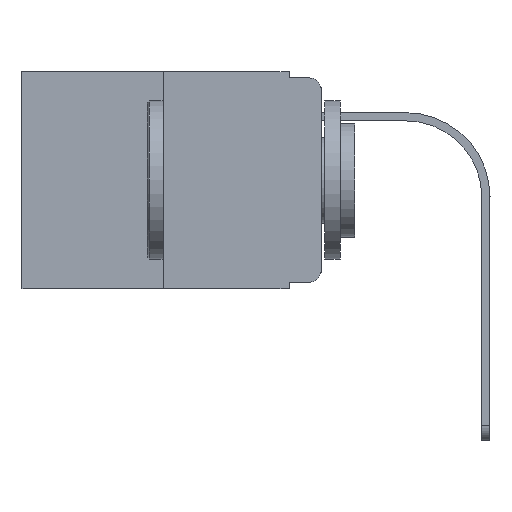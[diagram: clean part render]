
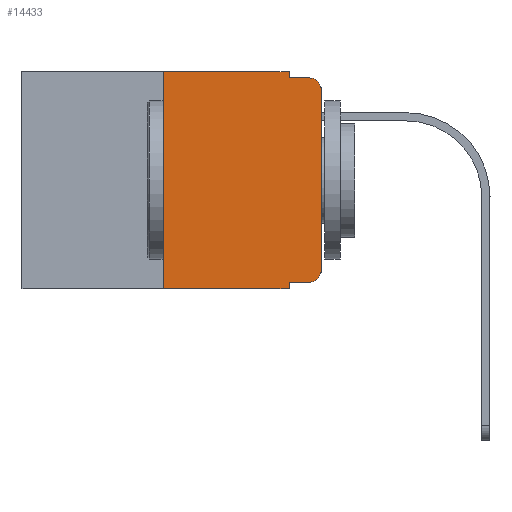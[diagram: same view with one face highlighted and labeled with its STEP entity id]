
A CAD part, left-side view. The second image highlights one B-rep face of the part: STEP entity #14433.
In plain terms, the highlighted planar face has unit normal (-1, 0, 0).
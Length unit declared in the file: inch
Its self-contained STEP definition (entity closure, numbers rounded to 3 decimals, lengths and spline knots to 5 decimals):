
#186 = CARTESIAN_POINT ( 'NONE',  ( 0., 0.051, -0.01 ) ) ;
#334 = CARTESIAN_POINT ( 'NONE',  ( 0., 0.02, -0.333 ) ) ;
#567 = DIRECTION ( 'NONE',  ( 0., -1., 0. ) ) ;
#605 = VECTOR ( 'NONE', #6141, 39.37008 ) ;
#712 = AXIS2_PLACEMENT_3D ( 'NONE', #1798, #9189, #21555 ) ;
#1086 = EDGE_CURVE ( 'NONE', #19642, #6668, #23073, .T. ) ;
#1165 = CARTESIAN_POINT ( 'NONE',  ( 0., 0.051, -0.01 ) ) ;
#1309 = CARTESIAN_POINT ( 'NONE',  ( 0., 0., -0.03 ) ) ;
#1361 = LINE ( 'NONE', #8524, #14861 ) ;
#1400 = ORIENTED_EDGE ( 'NONE', *, *, #13498, .F. ) ;
#1798 = CARTESIAN_POINT ( 'NONE',  ( 0., 0.02, -0.313 ) ) ;
#1829 = ORIENTED_EDGE ( 'NONE', *, *, #3514, .F. ) ;
#1975 = CARTESIAN_POINT ( 'NONE',  ( 0., 0.473, 0. ) ) ;
#2199 = EDGE_LOOP ( 'NONE', ( #4130, #20271, #1400, #1829, #14284, #20652, #4712, #16064, #18533, #12372 ) ) ;
#2959 = EDGE_CURVE ( 'NONE', #8968, #9520, #14927, .T. ) ;
#2961 = VECTOR ( 'NONE', #12769, 39.37008 ) ;
#3514 = EDGE_CURVE ( 'NONE', #9520, #6218, #1361, .T. ) ;
#3970 = CARTESIAN_POINT ( 'NONE',  ( 0., 0., 0. ) ) ;
#4130 = ORIENTED_EDGE ( 'NONE', *, *, #22395, .T. ) ;
#4528 = DIRECTION ( 'NONE',  ( 0., -1., 0. ) ) ;
#4606 = CARTESIAN_POINT ( 'NONE',  ( 0., 0.25, 0. ) ) ;
#4712 = ORIENTED_EDGE ( 'NONE', *, *, #4768, .T. ) ;
#4768 = EDGE_CURVE ( 'NONE', #12555, #6668, #19018, .T. ) ;
#5191 = EDGE_CURVE ( 'NONE', #19642, #13134, #20278, .T. ) ;
#6141 = DIRECTION ( 'NONE',  ( 0., -1., 0. ) ) ;
#6218 = VERTEX_POINT ( 'NONE', #1165 ) ;
#6524 = EDGE_CURVE ( 'NONE', #12555, #8968, #18800, .T. ) ;
#6668 = VERTEX_POINT ( 'NONE', #8411 ) ;
#6980 = DIRECTION ( 'NONE',  ( 0., 0., -1. ) ) ;
#7184 = DIRECTION ( 'NONE',  ( -1., 0., 0. ) ) ;
#7277 = FACE_OUTER_BOUND ( 'NONE', #2199, .T. ) ;
#8179 = CARTESIAN_POINT ( 'NONE',  ( 0., 0.473, -0.343 ) ) ;
#8202 = CIRCLE ( 'NONE', #11641, 0.02 ) ;
#8411 = CARTESIAN_POINT ( 'NONE',  ( 0., 0.051, -0.343 ) ) ;
#8524 = CARTESIAN_POINT ( 'NONE',  ( 0., 0.051, 0. ) ) ;
#8930 = CARTESIAN_POINT ( 'NONE',  ( 0., 0., -0.313 ) ) ;
#8968 = VERTEX_POINT ( 'NONE', #4606 ) ;
#9189 = DIRECTION ( 'NONE',  ( -1., 0., 0. ) ) ;
#9279 = DIRECTION ( 'NONE',  ( 0., 0., 1. ) ) ;
#9285 = PLANE ( 'NONE',  #16144 ) ;
#9520 = VERTEX_POINT ( 'NONE', #14572 ) ;
#10049 = CARTESIAN_POINT ( 'NONE',  ( 0., 0.25, -0.343 ) ) ;
#10499 = CARTESIAN_POINT ( 'NONE',  ( 0., 0.02, -0.03 ) ) ;
#11586 = CIRCLE ( 'NONE', #712, 0.02 ) ;
#11641 = AXIS2_PLACEMENT_3D ( 'NONE', #10499, #7184, #18031 ) ;
#12368 = DIRECTION ( 'NONE',  ( 0., 0., -1. ) ) ;
#12372 = ORIENTED_EDGE ( 'NONE', *, *, #19283, .T. ) ;
#12384 = DIRECTION ( 'NONE',  ( 0., 0., 1. ) ) ;
#12472 = CARTESIAN_POINT ( 'NONE',  ( 0., 0.051, -0.333 ) ) ;
#12555 = VERTEX_POINT ( 'NONE', #10049 ) ;
#12769 = DIRECTION ( 'NONE',  ( 0., -1., 0. ) ) ;
#12990 = LINE ( 'NONE', #186, #2961 ) ;
#13134 = VERTEX_POINT ( 'NONE', #334 ) ;
#13498 = EDGE_CURVE ( 'NONE', #6218, #17794, #12990, .T. ) ;
#13839 = CARTESIAN_POINT ( 'NONE',  ( 0., 0.25, 0. ) ) ;
#14284 = ORIENTED_EDGE ( 'NONE', *, *, #2959, .F. ) ;
#14433 = ADVANCED_FACE ( 'NONE', ( #7277 ), #9285, .F. ) ;
#14572 = CARTESIAN_POINT ( 'NONE',  ( 0., 0.051, 0. ) ) ;
#14861 = VECTOR ( 'NONE', #6980, 39.37008 ) ;
#14927 = LINE ( 'NONE', #1975, #16124 ) ;
#15494 = VECTOR ( 'NONE', #12384, 39.37008 ) ;
#15505 = DIRECTION ( 'NONE',  ( 1., 0., 0. ) ) ;
#15706 = VECTOR ( 'NONE', #12368, 39.37008 ) ;
#16064 = ORIENTED_EDGE ( 'NONE', *, *, #1086, .F. ) ;
#16124 = VECTOR ( 'NONE', #567, 39.37008 ) ;
#16144 = AXIS2_PLACEMENT_3D ( 'NONE', #19155, #15505, #22570 ) ;
#17794 = VERTEX_POINT ( 'NONE', #19221 ) ;
#18031 = DIRECTION ( 'NONE',  ( 0., 0., -1. ) ) ;
#18219 = LINE ( 'NONE', #3970, #19291 ) ;
#18533 = ORIENTED_EDGE ( 'NONE', *, *, #5191, .T. ) ;
#18800 = LINE ( 'NONE', #13839, #15494 ) ;
#19018 = LINE ( 'NONE', #8179, #20879 ) ;
#19155 = CARTESIAN_POINT ( 'NONE',  ( 0., 0.473, 0. ) ) ;
#19221 = CARTESIAN_POINT ( 'NONE',  ( 0., 0.02, -0.01 ) ) ;
#19283 = EDGE_CURVE ( 'NONE', #13134, #22273, #11586, .T. ) ;
#19291 = VECTOR ( 'NONE', #9279, 39.37008 ) ;
#19317 = CARTESIAN_POINT ( 'NONE',  ( 0., 0.051, 0. ) ) ;
#19485 = VERTEX_POINT ( 'NONE', #1309 ) ;
#19642 = VERTEX_POINT ( 'NONE', #12472 ) ;
#20271 = ORIENTED_EDGE ( 'NONE', *, *, #20474, .T. ) ;
#20278 = LINE ( 'NONE', #20637, #605 ) ;
#20474 = EDGE_CURVE ( 'NONE', #19485, #17794, #8202, .T. ) ;
#20637 = CARTESIAN_POINT ( 'NONE',  ( 0., 0.051, -0.333 ) ) ;
#20652 = ORIENTED_EDGE ( 'NONE', *, *, #6524, .F. ) ;
#20879 = VECTOR ( 'NONE', #4528, 39.37008 ) ;
#21555 = DIRECTION ( 'NONE',  ( 0., 0., -1. ) ) ;
#22273 = VERTEX_POINT ( 'NONE', #8930 ) ;
#22395 = EDGE_CURVE ( 'NONE', #22273, #19485, #18219, .T. ) ;
#22570 = DIRECTION ( 'NONE',  ( 0., 0., -1. ) ) ;
#23073 = LINE ( 'NONE', #19317, #15706 ) ;
